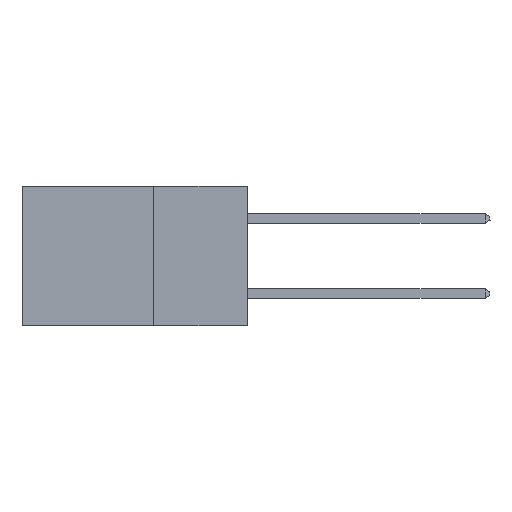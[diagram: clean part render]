
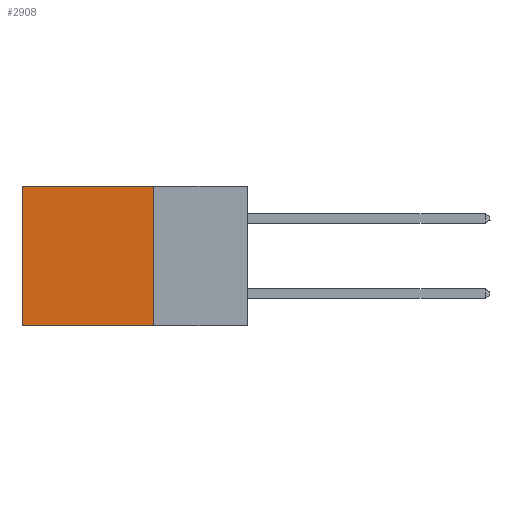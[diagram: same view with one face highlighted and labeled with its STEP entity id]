
A CAD part, left-side view. The second image highlights one B-rep face of the part: STEP entity #2908.
In plain terms, the highlighted planar face has unit normal (-1, 0, 0).
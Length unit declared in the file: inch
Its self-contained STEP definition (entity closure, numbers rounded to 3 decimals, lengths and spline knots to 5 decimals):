
#110 = EDGE_CURVE ( 'NONE', #20967, #28299, #15702, .T. ) ;
#279 = VERTEX_POINT ( 'NONE', #10387 ) ;
#1213 = CARTESIAN_POINT ( 'NONE',  ( 0.298, 0.25, 0. ) ) ;
#2908 = ADVANCED_FACE ( 'NONE', ( #4218 ), #8755, .F. ) ;
#4218 = FACE_OUTER_BOUND ( 'NONE', #15289, .T. ) ;
#5764 = EDGE_CURVE ( 'NONE', #279, #7426, #8095, .T. ) ;
#6057 = CARTESIAN_POINT ( 'NONE',  ( 0.298, 0.25, 0. ) ) ;
#7426 = VERTEX_POINT ( 'NONE', #9497 ) ;
#8095 = LINE ( 'NONE', #32981, #13800 ) ;
#8755 = PLANE ( 'NONE',  #26446 ) ;
#9080 = DIRECTION ( 'NONE',  ( 0., 0., -1. ) ) ;
#9497 = CARTESIAN_POINT ( 'NONE',  ( 0.298, 0.6, -0.37 ) ) ;
#10387 = CARTESIAN_POINT ( 'NONE',  ( 0.298, 0.6, 0. ) ) ;
#12456 = LINE ( 'NONE', #26075, #15288 ) ;
#13602 = ORIENTED_EDGE ( 'NONE', *, *, #5764, .T. ) ;
#13697 = CARTESIAN_POINT ( 'NONE',  ( 0.298, 0.25, -0.37 ) ) ;
#13800 = VECTOR ( 'NONE', #17270, 39.37008 ) ;
#15288 = VECTOR ( 'NONE', #31351, 39.37008 ) ;
#15289 = EDGE_LOOP ( 'NONE', ( #13602, #18774, #24732, #21472 ) ) ;
#15702 = LINE ( 'NONE', #1213, #25150 ) ;
#16287 = LINE ( 'NONE', #28482, #28592 ) ;
#16442 = DIRECTION ( 'NONE',  ( 1., 0., 0. ) ) ;
#17270 = DIRECTION ( 'NONE',  ( 0., 0., -1. ) ) ;
#18268 = EDGE_CURVE ( 'NONE', #28299, #7426, #12456, .T. ) ;
#18774 = ORIENTED_EDGE ( 'NONE', *, *, #18268, .F. ) ;
#20967 = VERTEX_POINT ( 'NONE', #6057 ) ;
#21472 = ORIENTED_EDGE ( 'NONE', *, *, #25596, .T. ) ;
#21541 = DIRECTION ( 'NONE',  ( 0., 0., -1. ) ) ;
#23435 = DIRECTION ( 'NONE',  ( 0., 1., 0. ) ) ;
#24732 = ORIENTED_EDGE ( 'NONE', *, *, #110, .F. ) ;
#25150 = VECTOR ( 'NONE', #9080, 39.37008 ) ;
#25596 = EDGE_CURVE ( 'NONE', #20967, #279, #16287, .T. ) ;
#26075 = CARTESIAN_POINT ( 'NONE',  ( 0.298, 0.25, -0.37 ) ) ;
#26446 = AXIS2_PLACEMENT_3D ( 'NONE', #27232, #16442, #21541 ) ;
#27232 = CARTESIAN_POINT ( 'NONE',  ( 0.298, 0.25, 0. ) ) ;
#28299 = VERTEX_POINT ( 'NONE', #13697 ) ;
#28482 = CARTESIAN_POINT ( 'NONE',  ( 0.298, 0.25, 0. ) ) ;
#28592 = VECTOR ( 'NONE', #23435, 39.37008 ) ;
#31351 = DIRECTION ( 'NONE',  ( 0., 1., 0. ) ) ;
#32981 = CARTESIAN_POINT ( 'NONE',  ( 0.298, 0.6, 0. ) ) ;
